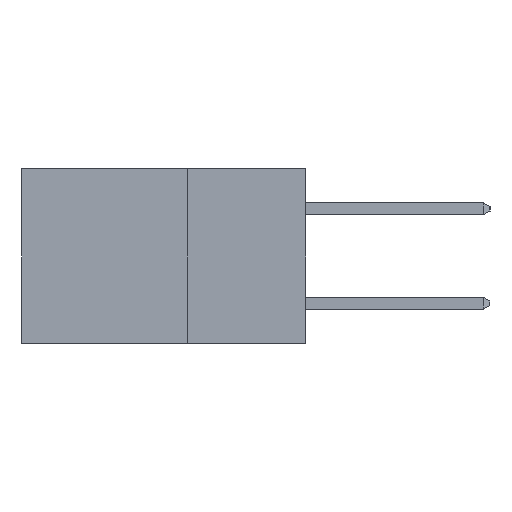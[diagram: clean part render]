
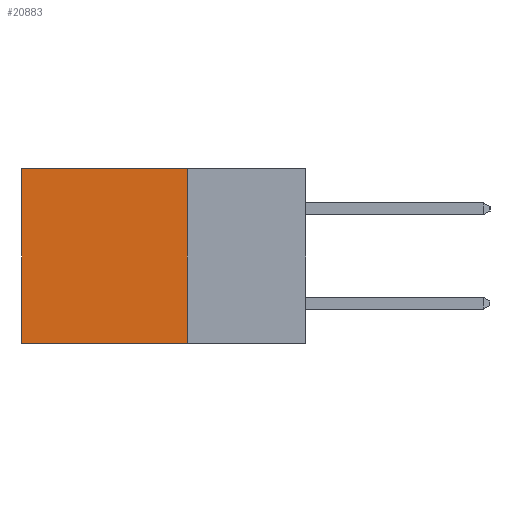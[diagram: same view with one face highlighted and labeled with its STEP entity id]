
A CAD part, left-side view. The second image highlights one B-rep face of the part: STEP entity #20883.
In plain terms, the highlighted planar face has unit normal (-1, 0, 0).
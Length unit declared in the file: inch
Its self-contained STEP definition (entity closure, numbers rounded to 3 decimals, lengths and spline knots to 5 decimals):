
#441 = VECTOR ( 'NONE', #11110, 39.37008 ) ;
#1143 = VERTEX_POINT ( 'NONE', #22031 ) ;
#2751 = VECTOR ( 'NONE', #13005, 39.37008 ) ;
#3147 = CARTESIAN_POINT ( 'NONE',  ( 0.2615, 0.25, -0.37 ) ) ;
#3165 = CARTESIAN_POINT ( 'NONE',  ( 0.2615, 0.25, -0.37 ) ) ;
#5240 = CARTESIAN_POINT ( 'NONE',  ( 0.2615, 0.25, -0.37 ) ) ;
#5334 = VECTOR ( 'NONE', #6752, 39.37008 ) ;
#5363 = ORIENTED_EDGE ( 'NONE', *, *, #18328, .F. ) ;
#5414 = AXIS2_PLACEMENT_3D ( 'NONE', #5240, #7006, #18980 ) ;
#6752 = DIRECTION ( 'NONE',  ( 0., 1., 0. ) ) ;
#7006 = DIRECTION ( 'NONE',  ( 1., 0., 0. ) ) ;
#8466 = DIRECTION ( 'NONE',  ( 0., 1., 0. ) ) ;
#8716 = VERTEX_POINT ( 'NONE', #13272 ) ;
#9413 = CARTESIAN_POINT ( 'NONE',  ( 0.2615, 0.25, -0.37 ) ) ;
#9950 = LINE ( 'NONE', #13534, #5334 ) ;
#11110 = DIRECTION ( 'NONE',  ( 0., 0., -1. ) ) ;
#11309 = CARTESIAN_POINT ( 'NONE',  ( 0.2615, 0.6, -0.37 ) ) ;
#12785 = ORIENTED_EDGE ( 'NONE', *, *, #15987, .T. ) ;
#13005 = DIRECTION ( 'NONE',  ( 0., 0., -1. ) ) ;
#13093 = VERTEX_POINT ( 'NONE', #3165 ) ;
#13272 = CARTESIAN_POINT ( 'NONE',  ( 0.2615, 0.25, 0. ) ) ;
#13534 = CARTESIAN_POINT ( 'NONE',  ( 0.2615, 0.25, 0. ) ) ;
#14128 = CARTESIAN_POINT ( 'NONE',  ( 0.2615, 0.6, -0.37 ) ) ;
#14337 = VERTEX_POINT ( 'NONE', #14128 ) ;
#14364 = LINE ( 'NONE', #9413, #441 ) ;
#14437 = VECTOR ( 'NONE', #8466, 39.37008 ) ;
#15493 = PLANE ( 'NONE',  #5414 ) ;
#15987 = EDGE_CURVE ( 'NONE', #8716, #1143, #9950, .T. ) ;
#16550 = LINE ( 'NONE', #11309, #2751 ) ;
#16971 = EDGE_CURVE ( 'NONE', #13093, #14337, #19019, .T. ) ;
#18328 = EDGE_CURVE ( 'NONE', #8716, #13093, #14364, .T. ) ;
#18533 = FACE_OUTER_BOUND ( 'NONE', #21900, .T. ) ;
#18980 = DIRECTION ( 'NONE',  ( 0., 0., -1. ) ) ;
#19019 = LINE ( 'NONE', #3147, #14437 ) ;
#19415 = ORIENTED_EDGE ( 'NONE', *, *, #22019, .T. ) ;
#19527 = ORIENTED_EDGE ( 'NONE', *, *, #16971, .F. ) ;
#20883 = ADVANCED_FACE ( 'NONE', ( #18533 ), #15493, .F. ) ;
#21900 = EDGE_LOOP ( 'NONE', ( #19415, #19527, #5363, #12785 ) ) ;
#22019 = EDGE_CURVE ( 'NONE', #1143, #14337, #16550, .T. ) ;
#22031 = CARTESIAN_POINT ( 'NONE',  ( 0.2615, 0.6, 0. ) ) ;
